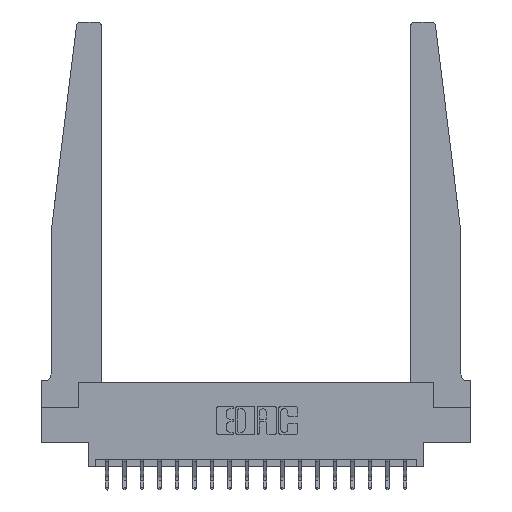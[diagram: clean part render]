
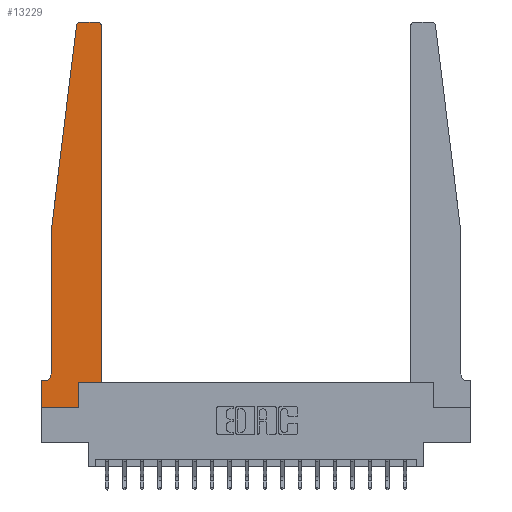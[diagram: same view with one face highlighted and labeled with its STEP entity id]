
A CAD part, top view. The second image highlights one B-rep face of the part: STEP entity #13229.
In plain terms, the highlighted planar face has unit normal (0, 0, 1).
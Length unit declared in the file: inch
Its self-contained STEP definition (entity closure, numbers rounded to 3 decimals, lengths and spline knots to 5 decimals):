
#160 = DIRECTION ( 'NONE',  ( 0., -1., 0. ) ) ;
#216 = DIRECTION ( 'NONE',  ( 1., 0., 0. ) ) ;
#344 = ORIENTED_EDGE ( 'NONE', *, *, #8770, .T. ) ;
#434 = AXIS2_PLACEMENT_3D ( 'NONE', #15052, #16612, #7303 ) ;
#528 = LINE ( 'NONE', #18835, #12973 ) ;
#600 = DIRECTION ( 'NONE',  ( 0., 0., 1. ) ) ;
#1043 = CARTESIAN_POINT ( 'NONE',  ( 0.065, 0.1875, 0.37 ) ) ;
#1134 = DIRECTION ( 'NONE',  ( 0., 0., 1. ) ) ;
#1792 = LINE ( 'NONE', #7937, #13746 ) ;
#2183 = ORIENTED_EDGE ( 'NONE', *, *, #15241, .T. ) ;
#2281 = VECTOR ( 'NONE', #17140, 39.37008 ) ;
#2642 = CARTESIAN_POINT ( 'NONE',  ( 0.425, 0.18, 0.37 ) ) ;
#2661 = FACE_OUTER_BOUND ( 'NONE', #16523, .T. ) ;
#2680 = CARTESIAN_POINT ( 'NONE',  ( 0.2605, 0.18, 0.37 ) ) ;
#2953 = LINE ( 'NONE', #2642, #15400 ) ;
#3623 = CARTESIAN_POINT ( 'NONE',  ( 0.2605, 0.18, 0.37 ) ) ;
#3826 = CARTESIAN_POINT ( 'NONE',  ( 0., 0., 0.37 ) ) ;
#3976 = ORIENTED_EDGE ( 'NONE', *, *, #9594, .T. ) ;
#4136 = PLANE ( 'NONE',  #434 ) ;
#4188 = EDGE_CURVE ( 'NONE', #9287, #9385, #17268, .T. ) ;
#4305 = LINE ( 'NONE', #9554, #15287 ) ;
#4466 = VECTOR ( 'NONE', #10458, 39.37008 ) ;
#4473 = EDGE_CURVE ( 'NONE', #12932, #18576, #4554, .T. ) ;
#4554 = CIRCLE ( 'NONE', #9497, 0.05 ) ;
#5037 = VERTEX_POINT ( 'NONE', #7142 ) ;
#5123 = CARTESIAN_POINT ( 'NONE',  ( 0.065, 0.2375, 0.37 ) ) ;
#5718 = CARTESIAN_POINT ( 'NONE',  ( 0.25, 2.75, 0.37 ) ) ;
#5814 = CARTESIAN_POINT ( 'NONE',  ( 0.425, 0.18, 0.37 ) ) ;
#5866 = CARTESIAN_POINT ( 'NONE',  ( 0.015, 0.2375, 0.37 ) ) ;
#5894 = AXIS2_PLACEMENT_3D ( 'NONE', #10481, #1134, #12038 ) ;
#6236 = CARTESIAN_POINT ( 'NONE',  ( 0.27653, 2.75, 0.37 ) ) ;
#6475 = LINE ( 'NONE', #7804, #2281 ) ;
#6510 = DIRECTION ( 'NONE',  ( 1., 0., 0. ) ) ;
#7142 = CARTESIAN_POINT ( 'NONE',  ( 0.395, 2.75, 0.37 ) ) ;
#7303 = DIRECTION ( 'NONE',  ( 1., 0., 0. ) ) ;
#7431 = DIRECTION ( 'NONE',  ( -1., 0., 0. ) ) ;
#7507 = VERTEX_POINT ( 'NONE', #19574 ) ;
#7582 = VERTEX_POINT ( 'NONE', #5814 ) ;
#7804 = CARTESIAN_POINT ( 'NONE',  ( 0.065, 1.25, 0.37 ) ) ;
#7886 = ORIENTED_EDGE ( 'NONE', *, *, #14922, .T. ) ;
#7937 = CARTESIAN_POINT ( 'NONE',  ( 0., 0., 0.37 ) ) ;
#7941 = CARTESIAN_POINT ( 'NONE',  ( 0., 0.1875, 0.37 ) ) ;
#8512 = ORIENTED_EDGE ( 'NONE', *, *, #4473, .T. ) ;
#8529 = EDGE_CURVE ( 'NONE', #16895, #5037, #14395, .T. ) ;
#8604 = LINE ( 'NONE', #1043, #4466 ) ;
#8731 = CARTESIAN_POINT ( 'NONE',  ( 0.425, 2.72, 0.37 ) ) ;
#8770 = EDGE_CURVE ( 'NONE', #18625, #11802, #17782, .T. ) ;
#9108 = ORIENTED_EDGE ( 'NONE', *, *, #10961, .T. ) ;
#9287 = VERTEX_POINT ( 'NONE', #11825 ) ;
#9385 = VERTEX_POINT ( 'NONE', #2680 ) ;
#9497 = AXIS2_PLACEMENT_3D ( 'NONE', #5866, #16748, #7431 ) ;
#9554 = CARTESIAN_POINT ( 'NONE',  ( 0., 0., 0.37 ) ) ;
#9567 = VECTOR ( 'NONE', #17770, 39.37008 ) ;
#9594 = EDGE_CURVE ( 'NONE', #7507, #12932, #6475, .T. ) ;
#9649 = EDGE_CURVE ( 'NONE', #16583, #9897, #1792, .T. ) ;
#9897 = VERTEX_POINT ( 'NONE', #3826 ) ;
#9925 = CARTESIAN_POINT ( 'NONE',  ( 0.24675, 2.72367, 0.37 ) ) ;
#9947 = CARTESIAN_POINT ( 'NONE',  ( 0.395, 2.72, 0.37 ) ) ;
#10458 = DIRECTION ( 'NONE',  ( -1., 0., 0. ) ) ;
#10481 = CARTESIAN_POINT ( 'NONE',  ( 0.27653, 2.72, 0.37 ) ) ;
#10612 = ORIENTED_EDGE ( 'NONE', *, *, #15876, .T. ) ;
#10961 = EDGE_CURVE ( 'NONE', #9385, #7582, #528, .T. ) ;
#11140 = EDGE_CURVE ( 'NONE', #11802, #7507, #18293, .T. ) ;
#11288 = EDGE_CURVE ( 'NONE', #7582, #16895, #2953, .T. ) ;
#11420 = ORIENTED_EDGE ( 'NONE', *, *, #4188, .T. ) ;
#11523 = DIRECTION ( 'NONE',  ( 1., 0., 0. ) ) ;
#11750 = ORIENTED_EDGE ( 'NONE', *, *, #9649, .T. ) ;
#11802 = VERTEX_POINT ( 'NONE', #9925 ) ;
#11825 = CARTESIAN_POINT ( 'NONE',  ( 0.2605, 0., 0.37 ) ) ;
#12038 = DIRECTION ( 'NONE',  ( 1., 0., 0. ) ) ;
#12535 = AXIS2_PLACEMENT_3D ( 'NONE', #9947, #600, #11523 ) ;
#12932 = VERTEX_POINT ( 'NONE', #5123 ) ;
#12973 = VECTOR ( 'NONE', #216, 39.37008 ) ;
#13229 = ADVANCED_FACE ( 'NONE', ( #2661 ), #4136, .T. ) ;
#13546 = DIRECTION ( 'NONE',  ( 0., 1., 0. ) ) ;
#13746 = VECTOR ( 'NONE', #160, 39.37008 ) ;
#14054 = LINE ( 'NONE', #5718, #18162 ) ;
#14395 = CIRCLE ( 'NONE', #12535, 0.03 ) ;
#14653 = CARTESIAN_POINT ( 'NONE',  ( 0.065, 1.25, 0.37 ) ) ;
#14656 = ORIENTED_EDGE ( 'NONE', *, *, #8529, .T. ) ;
#14791 = ORIENTED_EDGE ( 'NONE', *, *, #11140, .T. ) ;
#14922 = EDGE_CURVE ( 'NONE', #9897, #9287, #4305, .T. ) ;
#15043 = ORIENTED_EDGE ( 'NONE', *, *, #11288, .T. ) ;
#15044 = DIRECTION ( 'NONE',  ( -1., 0., 0. ) ) ;
#15052 = CARTESIAN_POINT ( 'NONE',  ( 0., 0.1875, 0.37 ) ) ;
#15241 = EDGE_CURVE ( 'NONE', #5037, #18625, #14054, .T. ) ;
#15287 = VECTOR ( 'NONE', #6510, 39.37008 ) ;
#15400 = VECTOR ( 'NONE', #13546, 39.37008 ) ;
#15876 = EDGE_CURVE ( 'NONE', #18576, #16583, #8604, .T. ) ;
#16523 = EDGE_LOOP ( 'NONE', ( #2183, #344, #14791, #3976, #8512, #10612, #11750, #7886, #11420, #9108, #15043, #14656 ) ) ;
#16583 = VERTEX_POINT ( 'NONE', #7941 ) ;
#16612 = DIRECTION ( 'NONE',  ( 0., 0., 1. ) ) ;
#16746 = VECTOR ( 'NONE', #17641, 39.37008 ) ;
#16748 = DIRECTION ( 'NONE',  ( 0., 0., -1. ) ) ;
#16895 = VERTEX_POINT ( 'NONE', #8731 ) ;
#17140 = DIRECTION ( 'NONE',  ( 0., -1., 0. ) ) ;
#17268 = LINE ( 'NONE', #3623, #16746 ) ;
#17641 = DIRECTION ( 'NONE',  ( 0., 1., 0. ) ) ;
#17770 = DIRECTION ( 'NONE',  ( -0.122, -0.992, 0. ) ) ;
#17782 = CIRCLE ( 'NONE', #5894, 0.03 ) ;
#18162 = VECTOR ( 'NONE', #15044, 39.37008 ) ;
#18293 = LINE ( 'NONE', #14653, #9567 ) ;
#18576 = VERTEX_POINT ( 'NONE', #20036 ) ;
#18625 = VERTEX_POINT ( 'NONE', #6236 ) ;
#18835 = CARTESIAN_POINT ( 'NONE',  ( 0.425, 0.18, 0.37 ) ) ;
#19574 = CARTESIAN_POINT ( 'NONE',  ( 0.065, 1.25, 0.37 ) ) ;
#20036 = CARTESIAN_POINT ( 'NONE',  ( 0.015, 0.1875, 0.37 ) ) ;
